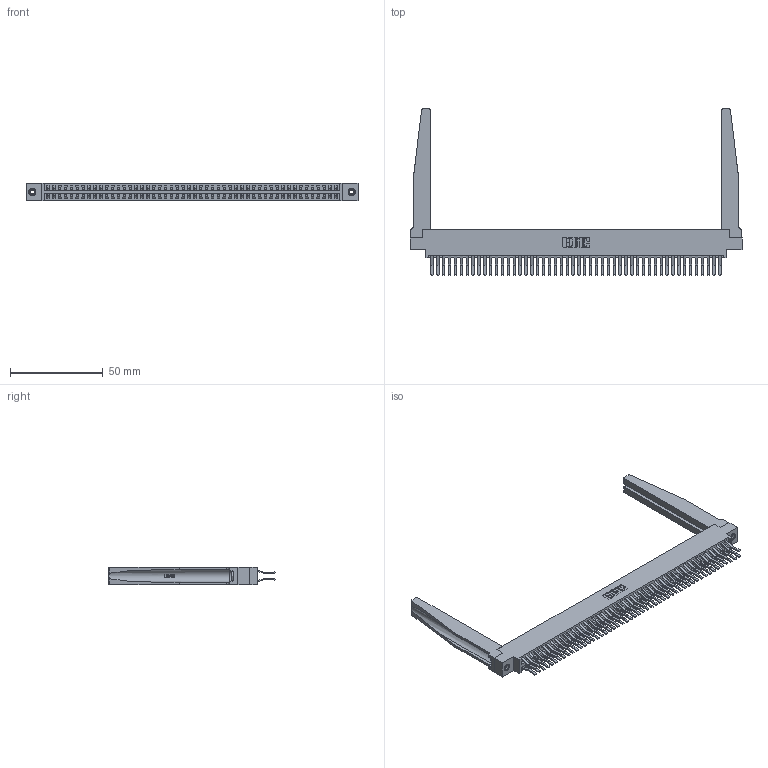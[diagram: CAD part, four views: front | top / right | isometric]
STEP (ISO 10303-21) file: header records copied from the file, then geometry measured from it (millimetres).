
FILE_DESCRIPTION (( 'STEP AP203' ), '1' );
FILE_NAME ('346-100-560-878.STEP', '2022-05-26T21:54:41', ( '' ), ( '' ), 'SwSTEP 2.0', 'SolidWorks 2020', '' );
FILE_SCHEMA (( 'CONFIG_CONTROL_DESIGN' ));
Length unit declared in the file: inch
Products named in the file (5): 346-100-560-878; 346-220-078_345-220-078; 345-292-001_560 Tail; 345-250-001_345-250-001-102; 346 Part_0.170 Offset - 0.156 Dia-TH
Assembly tree (105 placements, depth 2):
  346-100-560-878
    346 Part_0.170 Offset - 0.156 Dia-TH
    345-292-001_560 Tail  x100
    346-220-078_345-220-078  x2
    345-250-001_345-250-001-102  x2
Bounding box: 179.32 x 90.05 x 9.4 mm (x, y, z)
Volume: 24940.1 mm3; surface area: 33411.3 mm2
Topology: 105 solids, 105 shells, 5774 faces, 17085 edges, 11246 vertices
Faces by surface type: plane 3736, cylinder 1986, bspline 36, cone 12, torus 4
Entity records: 36938 total; most frequent: CARTESIAN_POINT 7021, ORIENTED_EDGE 5842, DIRECTION 5227, EDGE_CURVE 2921, LINE 2491, VECTOR 2491, VERTEX_POINT 1940, AXIS2_PLACEMENT_3D 1368
